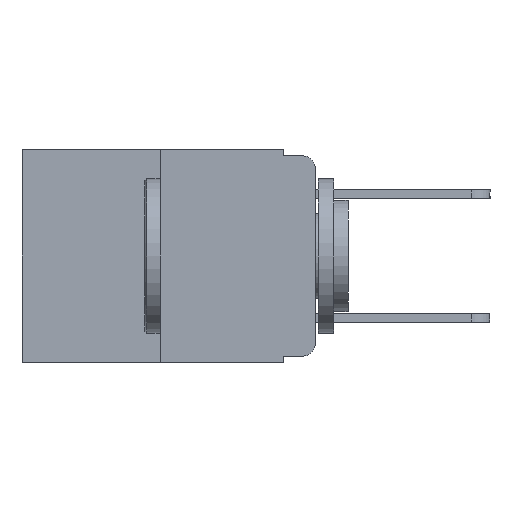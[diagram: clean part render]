
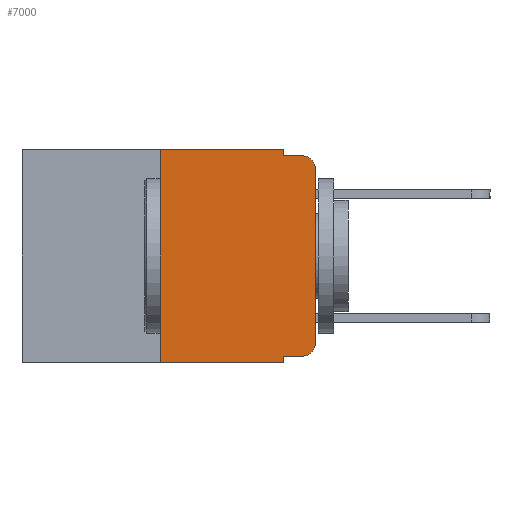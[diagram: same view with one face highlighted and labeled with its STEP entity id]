
A CAD part, left-side view. The second image highlights one B-rep face of the part: STEP entity #7000.
In plain terms, the highlighted planar face has unit normal (-1, 0, 0).
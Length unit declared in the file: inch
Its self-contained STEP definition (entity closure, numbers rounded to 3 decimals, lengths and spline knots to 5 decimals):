
#185 = VERTEX_POINT ( 'NONE', #7240 ) ;
#191 = CARTESIAN_POINT ( 'NONE',  ( 0., 0.051, -0.333 ) ) ;
#494 = PLANE ( 'NONE',  #8556 ) ;
#533 = DIRECTION ( 'NONE',  ( 0., -1., 0. ) ) ;
#1186 = CARTESIAN_POINT ( 'NONE',  ( 0., 0.473, 0. ) ) ;
#1478 = VECTOR ( 'NONE', #13445, 39.37008 ) ;
#1696 = CARTESIAN_POINT ( 'NONE',  ( 0., 0., -0.313 ) ) ;
#1722 = CARTESIAN_POINT ( 'NONE',  ( 0., 0.051, 0. ) ) ;
#1744 = DIRECTION ( 'NONE',  ( 0., 0., 1. ) ) ;
#1821 = CARTESIAN_POINT ( 'NONE',  ( 0., 0.473, 0. ) ) ;
#1886 = CARTESIAN_POINT ( 'NONE',  ( 0., 0.473, -0.343 ) ) ;
#1905 = VECTOR ( 'NONE', #533, 39.37008 ) ;
#1924 = LINE ( 'NONE', #1722, #12945 ) ;
#1981 = VERTEX_POINT ( 'NONE', #6950 ) ;
#2159 = DIRECTION ( 'NONE',  ( -1., 0., 0. ) ) ;
#2212 = VERTEX_POINT ( 'NONE', #5918 ) ;
#2320 = LINE ( 'NONE', #6837, #7985 ) ;
#2438 = DIRECTION ( 'NONE',  ( 0., -1., 0. ) ) ;
#2982 = CARTESIAN_POINT ( 'NONE',  ( 0., 0.051, 0. ) ) ;
#3087 = VECTOR ( 'NONE', #2438, 39.37008 ) ;
#3102 = VERTEX_POINT ( 'NONE', #1696 ) ;
#3119 = EDGE_CURVE ( 'NONE', #1981, #4566, #7635, .T. ) ;
#3829 = LINE ( 'NONE', #4311, #3087 ) ;
#4311 = CARTESIAN_POINT ( 'NONE',  ( 0., 0.051, -0.333 ) ) ;
#4328 = VERTEX_POINT ( 'NONE', #12259 ) ;
#4329 = AXIS2_PLACEMENT_3D ( 'NONE', #13722, #2159, #10317 ) ;
#4515 = LINE ( 'NONE', #1886, #12141 ) ;
#4566 = VERTEX_POINT ( 'NONE', #2982 ) ;
#4914 = DIRECTION ( 'NONE',  ( 0., -1., 0. ) ) ;
#4950 = ORIENTED_EDGE ( 'NONE', *, *, #7523, .T. ) ;
#5101 = CIRCLE ( 'NONE', #5862, 0.02 ) ;
#5245 = VERTEX_POINT ( 'NONE', #13810 ) ;
#5443 = ORIENTED_EDGE ( 'NONE', *, *, #7666, .T. ) ;
#5450 = LINE ( 'NONE', #10359, #13278 ) ;
#5481 = DIRECTION ( 'NONE',  ( 0., -1., 0. ) ) ;
#5562 = ORIENTED_EDGE ( 'NONE', *, *, #7668, .T. ) ;
#5642 = ORIENTED_EDGE ( 'NONE', *, *, #7529, .T. ) ;
#5673 = ORIENTED_EDGE ( 'NONE', *, *, #7623, .F. ) ;
#5785 = LINE ( 'NONE', #10066, #10645 ) ;
#5862 = AXIS2_PLACEMENT_3D ( 'NONE', #12451, #6173, #13882 ) ;
#5918 = CARTESIAN_POINT ( 'NONE',  ( 0., 0.051, -0.343 ) ) ;
#6119 = DIRECTION ( 'NONE',  ( 0., 0., -1. ) ) ;
#6173 = DIRECTION ( 'NONE',  ( -1., 0., 0. ) ) ;
#6323 = VERTEX_POINT ( 'NONE', #191 ) ;
#6837 = CARTESIAN_POINT ( 'NONE',  ( 0., 0.25, 0. ) ) ;
#6950 = CARTESIAN_POINT ( 'NONE',  ( 0., 0.25, 0. ) ) ;
#7000 = ADVANCED_FACE ( 'NONE', ( #10362 ), #494, .F. ) ;
#7146 = ORIENTED_EDGE ( 'NONE', *, *, #8199, .T. ) ;
#7240 = CARTESIAN_POINT ( 'NONE',  ( 0., 0.25, -0.343 ) ) ;
#7523 = EDGE_CURVE ( 'NONE', #4328, #3102, #8975, .T. ) ;
#7529 = EDGE_CURVE ( 'NONE', #6323, #4328, #3829, .T. ) ;
#7623 = EDGE_CURVE ( 'NONE', #6323, #2212, #5450, .T. ) ;
#7624 = EDGE_CURVE ( 'NONE', #185, #1981, #2320, .T. ) ;
#7635 = LINE ( 'NONE', #1821, #1905 ) ;
#7641 = EDGE_CURVE ( 'NONE', #4566, #14083, #1924, .T. ) ;
#7647 = EDGE_CURVE ( 'NONE', #14083, #8126, #5785, .T. ) ;
#7666 = EDGE_CURVE ( 'NONE', #5245, #8126, #5101, .T. ) ;
#7668 = EDGE_CURVE ( 'NONE', #3102, #5245, #10347, .T. ) ;
#7698 = ORIENTED_EDGE ( 'NONE', *, *, #7647, .F. ) ;
#7985 = VECTOR ( 'NONE', #1744, 39.37008 ) ;
#8126 = VERTEX_POINT ( 'NONE', #8533 ) ;
#8199 = EDGE_CURVE ( 'NONE', #185, #2212, #4515, .T. ) ;
#8533 = CARTESIAN_POINT ( 'NONE',  ( 0., 0.02, -0.01 ) ) ;
#8556 = AXIS2_PLACEMENT_3D ( 'NONE', #1186, #13326, #12135 ) ;
#8975 = CIRCLE ( 'NONE', #4329, 0.02 ) ;
#9131 = CARTESIAN_POINT ( 'NONE',  ( 0., 0.051, -0.01 ) ) ;
#9429 = ORIENTED_EDGE ( 'NONE', *, *, #7624, .F. ) ;
#10066 = CARTESIAN_POINT ( 'NONE',  ( 0., 0.051, -0.01 ) ) ;
#10317 = DIRECTION ( 'NONE',  ( 0., 0., -1. ) ) ;
#10347 = LINE ( 'NONE', #13481, #1478 ) ;
#10359 = CARTESIAN_POINT ( 'NONE',  ( 0., 0.051, 0. ) ) ;
#10362 = FACE_OUTER_BOUND ( 'NONE', #11698, .T. ) ;
#10645 = VECTOR ( 'NONE', #4914, 39.37008 ) ;
#11071 = ORIENTED_EDGE ( 'NONE', *, *, #7641, .F. ) ;
#11215 = ORIENTED_EDGE ( 'NONE', *, *, #3119, .F. ) ;
#11698 = EDGE_LOOP ( 'NONE', ( #5562, #5443, #7698, #11071, #11215, #9429, #7146, #5673, #5642, #4950 ) ) ;
#12135 = DIRECTION ( 'NONE',  ( 0., 0., -1. ) ) ;
#12141 = VECTOR ( 'NONE', #5481, 39.37008 ) ;
#12259 = CARTESIAN_POINT ( 'NONE',  ( 0., 0.02, -0.333 ) ) ;
#12451 = CARTESIAN_POINT ( 'NONE',  ( 0., 0.02, -0.03 ) ) ;
#12945 = VECTOR ( 'NONE', #13289, 39.37008 ) ;
#13278 = VECTOR ( 'NONE', #6119, 39.37008 ) ;
#13289 = DIRECTION ( 'NONE',  ( 0., 0., -1. ) ) ;
#13326 = DIRECTION ( 'NONE',  ( 1., 0., 0. ) ) ;
#13445 = DIRECTION ( 'NONE',  ( 0., 0., 1. ) ) ;
#13481 = CARTESIAN_POINT ( 'NONE',  ( 0., 0., 0. ) ) ;
#13722 = CARTESIAN_POINT ( 'NONE',  ( 0., 0.02, -0.313 ) ) ;
#13810 = CARTESIAN_POINT ( 'NONE',  ( 0., 0., -0.03 ) ) ;
#13882 = DIRECTION ( 'NONE',  ( 0., 0., -1. ) ) ;
#14083 = VERTEX_POINT ( 'NONE', #9131 ) ;
